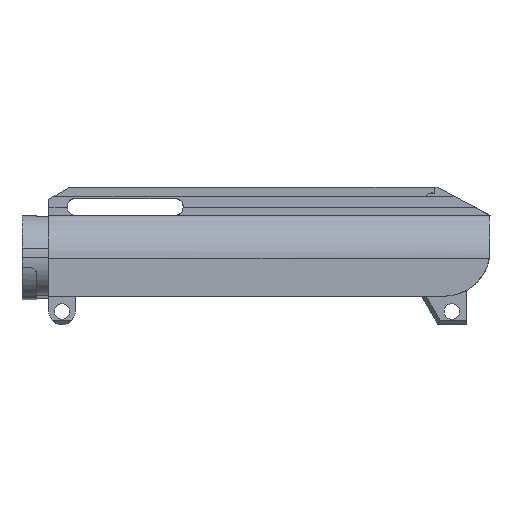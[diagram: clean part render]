
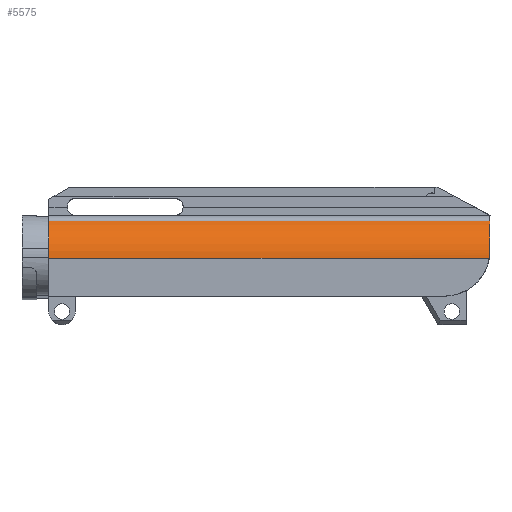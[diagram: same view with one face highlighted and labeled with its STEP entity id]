
A CAD part, top view. The second image highlights one B-rep face of the part: STEP entity #5575.
In plain terms, the highlighted cylindrical face has radius 18.582 mm (diameter 37.163 mm), a partial arc.
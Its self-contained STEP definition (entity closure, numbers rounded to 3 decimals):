
#72 = ORIENTED_EDGE ( 'NONE', *, *, #1827, .T. ) ;
#402 = VERTEX_POINT ( 'NONE', #4501 ) ;
#529 = ORIENTED_EDGE ( 'NONE', *, *, #8859, .T. ) ;
#771 = DIRECTION ( 'NONE',  ( 0., 1., 0. ) ) ;
#873 = CARTESIAN_POINT ( 'NONE',  ( 202.949, -122.426, -11.312 ) ) ;
#947 = CARTESIAN_POINT ( 'NONE',  ( 202.949, -137.993, -2.071 ) ) ;
#960 = DIRECTION ( 'NONE',  ( 1., 0., 0. ) ) ;
#1399 = DIRECTION ( 'NONE',  ( 1., 0., 0. ) ) ;
#1522 = VERTEX_POINT ( 'NONE', #8615 ) ;
#1639 = LINE ( 'NONE', #873, #9458 ) ;
#1649 = VERTEX_POINT ( 'NONE', #8036 ) ;
#1827 = EDGE_CURVE ( 'NONE', #6430, #1649, #1960, .T. ) ;
#1869 = CARTESIAN_POINT ( 'NONE',  ( 397.354, -136.851, -2.102 ) ) ;
#1884 = EDGE_CURVE ( 'NONE', #4789, #402, #5351, .T. ) ;
#1960 = CIRCLE ( 'NONE', #3803, 18.582 ) ;
#1986 = EDGE_CURVE ( 'NONE', #402, #2139, #3124, .T. ) ;
#2122 = ORIENTED_EDGE ( 'NONE', *, *, #1986, .T. ) ;
#2139 = VERTEX_POINT ( 'NONE', #6884 ) ;
#2177 = AXIS2_PLACEMENT_3D ( 'NONE', #7529, #960, #771 ) ;
#2575 = CARTESIAN_POINT ( 'NONE',  ( 397.354, -138.493, -20.646 ) ) ;
#2650 = CARTESIAN_POINT ( 'NONE',  ( 397.353, -135.717, -2.237 ) ) ;
#2889 = AXIS2_PLACEMENT_3D ( 'NONE', #7830, #4156, #3523 ) ;
#3124 = LINE ( 'NONE', #947, #6278 ) ;
#3216 = CARTESIAN_POINT ( 'NONE',  ( 397.049, -137.993, -2.071 ) ) ;
#3462 = CARTESIAN_POINT ( 'NONE',  ( 397.353, -134.6, -2.477 ) ) ;
#3523 = DIRECTION ( 'NONE',  ( 0., 0., 1. ) ) ;
#3803 = AXIS2_PLACEMENT_3D ( 'NONE', #2575, #7589, #6143 ) ;
#4156 = DIRECTION ( 'NONE',  ( 1., 0., 0. ) ) ;
#4501 = CARTESIAN_POINT ( 'NONE',  ( 214.061, -137.993, -2.071 ) ) ;
#4559 = CARTESIAN_POINT ( 'NONE',  ( 214.061, -122.426, -11.312 ) ) ;
#4789 = VERTEX_POINT ( 'NONE', #4559 ) ;
#4861 = CARTESIAN_POINT ( 'NONE',  ( 397.354, -137.993, -2.071 ) ) ;
#5351 = CIRCLE ( 'NONE', #2889, 18.582 ) ;
#5575 = ADVANCED_FACE ( 'NONE', ( #8890 ), #7441, .T. ) ;
#5796 = EDGE_LOOP ( 'NONE', ( #72, #8732, #8643, #2122, #6276, #529 ) ) ;
#6143 = DIRECTION ( 'NONE',  ( 0., 1., 0. ) ) ;
#6178 = CARTESIAN_POINT ( 'NONE',  ( 397.354, -137.993, -2.071 ) ) ;
#6276 = ORIENTED_EDGE ( 'NONE', *, *, #9049, .T. ) ;
#6278 = VECTOR ( 'NONE', #1399, 1000. ) ;
#6430 = VERTEX_POINT ( 'NONE', #6178 ) ;
#6469 = B_SPLINE_CURVE_WITH_KNOTS ( 'NONE', 3,
 ( #3216, #9151, #8332, #8381 ),
 .UNSPECIFIED., .F., .F.,
 ( 4, 4 ),
 ( 0., 0.003 ),
 .UNSPECIFIED. ) ;
#6884 = CARTESIAN_POINT ( 'NONE',  ( 397.049, -137.993, -2.071 ) ) ;
#7191 =( BOUNDED_CURVE ( )  B_SPLINE_CURVE ( 3, ( #3462, #2650, #1869, #4861 ),
 .UNSPECIFIED., .F., .T. ) 
 B_SPLINE_CURVE_WITH_KNOTS ( ( 4, 4 ),
 ( 4.501, 4.685 ),
 .UNSPECIFIED. ) 
 CURVE ( )  GEOMETRIC_REPRESENTATION_ITEM ( )  RATIONAL_B_SPLINE_CURVE ( ( 1., 0.997, 0.997, 1. ) ) 
 REPRESENTATION_ITEM ( '' )  );
#7441 = CYLINDRICAL_SURFACE ( 'NONE', #2177, 18.582 ) ;
#7529 = CARTESIAN_POINT ( 'NONE',  ( 202.949, -138.493, -20.646 ) ) ;
#7589 = DIRECTION ( 'NONE',  ( -1., 0., 0. ) ) ;
#7830 = CARTESIAN_POINT ( 'NONE',  ( 214.061, -138.493, -20.646 ) ) ;
#8017 = EDGE_CURVE ( 'NONE', #1649, #4789, #1639, .T. ) ;
#8036 = CARTESIAN_POINT ( 'NONE',  ( 397.354, -122.426, -11.312 ) ) ;
#8332 = CARTESIAN_POINT ( 'NONE',  ( 397.353, -135.728, -2.235 ) ) ;
#8381 = CARTESIAN_POINT ( 'NONE',  ( 397.353, -134.6, -2.477 ) ) ;
#8615 = CARTESIAN_POINT ( 'NONE',  ( 397.353, -134.6, -2.477 ) ) ;
#8643 = ORIENTED_EDGE ( 'NONE', *, *, #1884, .T. ) ;
#8732 = ORIENTED_EDGE ( 'NONE', *, *, #8017, .T. ) ;
#8859 = EDGE_CURVE ( 'NONE', #1522, #6430, #7191, .T. ) ;
#8890 = FACE_OUTER_BOUND ( 'NONE', #5796, .T. ) ;
#9049 = EDGE_CURVE ( 'NONE', #2139, #1522, #6469, .T. ) ;
#9151 = CARTESIAN_POINT ( 'NONE',  ( 397.254, -136.859, -2.101 ) ) ;
#9435 = DIRECTION ( 'NONE',  ( -1., 0., 0. ) ) ;
#9458 = VECTOR ( 'NONE', #9435, 1000. ) ;
